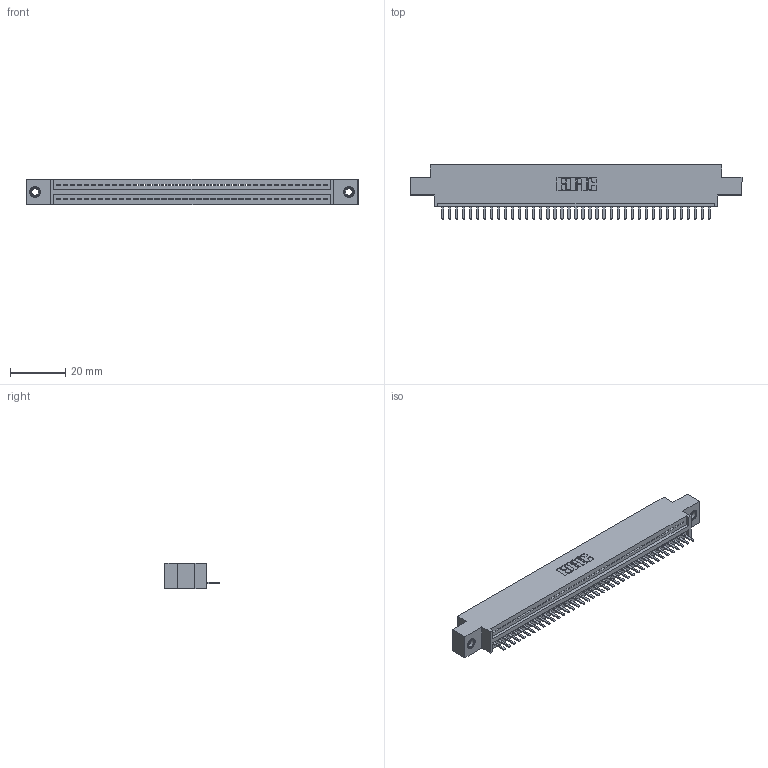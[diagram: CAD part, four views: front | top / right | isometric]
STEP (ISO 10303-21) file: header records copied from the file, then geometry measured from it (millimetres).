
FILE_DESCRIPTION (( 'STEP AP203' ), '1' );
FILE_NAME ('345-039-520-607.STEP', '2018-08-30T11:35:36', ( '' ), ( '' ), 'SwSTEP 2.0', 'SolidWorks 2016', '' );
FILE_SCHEMA (( 'CONFIG_CONTROL_DESIGN' ));
Length unit declared in the file: inch
Products named in the file (4): 345-250-001_345-250-005-103; 345-039-520-607; 345 Part_0.170 Offset - 0.156 Dia-TI; 345-292-001_345-293-120
Assembly tree (42 placements, depth 2):
  345-039-520-607
    345 Part_0.170 Offset - 0.156 Dia-TI
    345-292-001_345-293-120  x39
    345-250-001_345-250-005-103  x2
Bounding box: 120.27 x 19.68 x 9.4 mm (x, y, z)
Volume: 11159.6 mm3; surface area: 14581.4 mm2
Topology: 42 solids, 42 shells, 2608 faces, 7665 edges, 4998 vertices
Faces by surface type: plane 1754, cylinder 838, cone 12, torus 4
Entity records: 31188 total; most frequent: CARTESIAN_POINT 5396, ORIENTED_EDGE 5350, DIRECTION 4731, EDGE_CURVE 2675, VECTOR 2363, LINE 2363, VERTEX_POINT 1776, AXIS2_PLACEMENT_3D 1184
